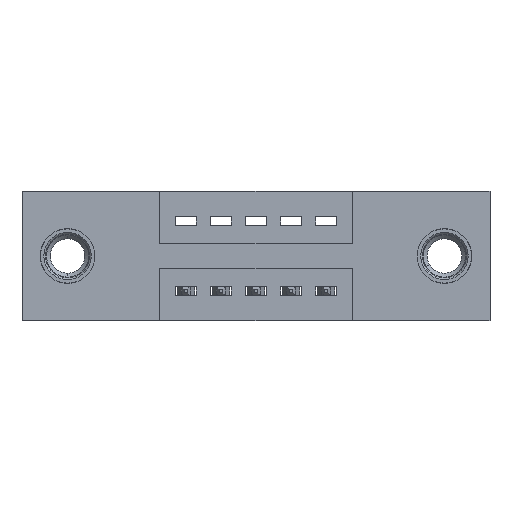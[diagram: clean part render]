
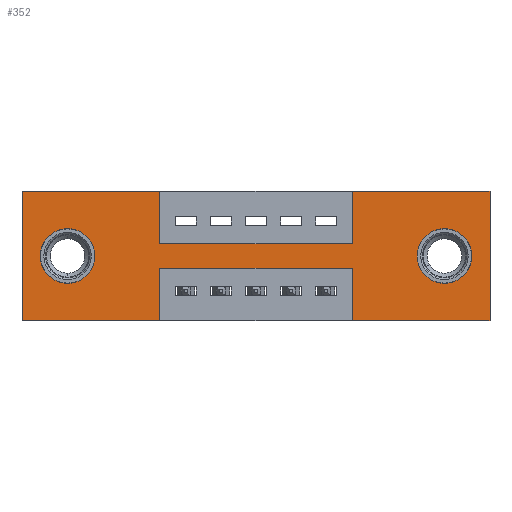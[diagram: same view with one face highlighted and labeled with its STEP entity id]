
A CAD part, front view. The second image highlights one B-rep face of the part: STEP entity #352.
In plain terms, the highlighted planar face has unit normal (0, -1, 0).
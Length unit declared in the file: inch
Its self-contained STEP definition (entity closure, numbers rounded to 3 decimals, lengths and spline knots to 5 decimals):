
#28 = VERTEX_POINT ( 'NONE', #2051 ) ;
#45 = CARTESIAN_POINT ( 'NONE',  ( 0.13, 0., -0.263 ) ) ;
#69 = ORIENTED_EDGE ( 'NONE', *, *, #4943, .F. ) ;
#73 = CARTESIAN_POINT ( 'NONE',  ( 0.3925, 0., -0.22 ) ) ;
#151 = VECTOR ( 'NONE', #3719, 39.37008 ) ;
#238 = CIRCLE ( 'NONE', #2748, 0.078 ) ;
#253 = VERTEX_POINT ( 'NONE', #2295 ) ;
#296 = CARTESIAN_POINT ( 'NONE',  ( 0.9425, 0., -0.37 ) ) ;
#352 = ADVANCED_FACE ( 'NONE', ( #1075, #2657, #8545 ), #2574, .T. ) ;
#358 = DIRECTION ( 'NONE',  ( 0., 0., -1. ) ) ;
#385 = VECTOR ( 'NONE', #1901, 39.37008 ) ;
#388 = VERTEX_POINT ( 'NONE', #4144 ) ;
#391 = DIRECTION ( 'NONE',  ( 0., 1., 0. ) ) ;
#530 = CARTESIAN_POINT ( 'NONE',  ( 0., 0., 0. ) ) ;
#558 = ORIENTED_EDGE ( 'NONE', *, *, #7253, .F. ) ;
#677 = VERTEX_POINT ( 'NONE', #1486 ) ;
#724 = LINE ( 'NONE', #1083, #8659 ) ;
#763 = VERTEX_POINT ( 'NONE', #45 ) ;
#806 = EDGE_CURVE ( 'NONE', #6764, #9784, #9596, .T. ) ;
#897 = CARTESIAN_POINT ( 'NONE',  ( 0.9425, 0., -0.15 ) ) ;
#1017 = DIRECTION ( 'NONE',  ( 0., 1., 0. ) ) ;
#1075 = FACE_BOUND ( 'NONE', #9132, .T. ) ;
#1083 = CARTESIAN_POINT ( 'NONE',  ( 1.335, 0., 0. ) ) ;
#1161 = ORIENTED_EDGE ( 'NONE', *, *, #9936, .F. ) ;
#1311 = VECTOR ( 'NONE', #2848, 39.37008 ) ;
#1486 = CARTESIAN_POINT ( 'NONE',  ( 1.205, 0., -0.107 ) ) ;
#1519 = ORIENTED_EDGE ( 'NONE', *, *, #2646, .F. ) ;
#1689 = LINE ( 'NONE', #6622, #5792 ) ;
#1882 = EDGE_LOOP ( 'NONE', ( #9166, #5014 ) ) ;
#1901 = DIRECTION ( 'NONE',  ( 1., 0., 0. ) ) ;
#1943 = LINE ( 'NONE', #9432, #7854 ) ;
#2003 = DIRECTION ( 'NONE',  ( 0., 0., 1. ) ) ;
#2026 = EDGE_CURVE ( 'NONE', #4399, #3299, #5590, .T. ) ;
#2037 = CARTESIAN_POINT ( 'NONE',  ( 0.3925, 0., -0.22 ) ) ;
#2051 = CARTESIAN_POINT ( 'NONE',  ( 0., 0., 0. ) ) ;
#2217 = LINE ( 'NONE', #296, #5832 ) ;
#2295 = CARTESIAN_POINT ( 'NONE',  ( 0.3925, 0., -0.15 ) ) ;
#2343 = VECTOR ( 'NONE', #5898, 39.37008 ) ;
#2426 = AXIS2_PLACEMENT_3D ( 'NONE', #8633, #4018, #9411 ) ;
#2428 = LINE ( 'NONE', #3425, #385 ) ;
#2490 = EDGE_CURVE ( 'NONE', #3299, #6764, #2217, .T. ) ;
#2574 = PLANE ( 'NONE',  #4707 ) ;
#2646 = EDGE_CURVE ( 'NONE', #6790, #7220, #8218, .T. ) ;
#2657 = FACE_BOUND ( 'NONE', #1882, .T. ) ;
#2668 = ORIENTED_EDGE ( 'NONE', *, *, #2026, .F. ) ;
#2745 = CARTESIAN_POINT ( 'NONE',  ( 0.9425, 0., -0.22 ) ) ;
#2748 = AXIS2_PLACEMENT_3D ( 'NONE', #4505, #9869, #5278 ) ;
#2848 = DIRECTION ( 'NONE',  ( -1., 0., 0. ) ) ;
#2850 = DIRECTION ( 'NONE',  ( -1., 0., 0. ) ) ;
#2927 = DIRECTION ( 'NONE',  ( -1., 0., 0. ) ) ;
#2999 = CIRCLE ( 'NONE', #9255, 0.078 ) ;
#3002 = EDGE_CURVE ( 'NONE', #763, #7161, #5111, .T. ) ;
#3026 = VECTOR ( 'NONE', #7493, 39.37008 ) ;
#3113 = ORIENTED_EDGE ( 'NONE', *, *, #4384, .F. ) ;
#3299 = VERTEX_POINT ( 'NONE', #9014 ) ;
#3335 = DIRECTION ( 'NONE',  ( 0., -1., 0. ) ) ;
#3425 = CARTESIAN_POINT ( 'NONE',  ( 0.3925, 0., -0.15 ) ) ;
#3529 = ORIENTED_EDGE ( 'NONE', *, *, #4447, .F. ) ;
#3543 = VECTOR ( 'NONE', #2927, 39.37008 ) ;
#3552 = CARTESIAN_POINT ( 'NONE',  ( 1.335, 0., -0.37 ) ) ;
#3719 = DIRECTION ( 'NONE',  ( 1., 0., 0. ) ) ;
#3785 = CARTESIAN_POINT ( 'NONE',  ( 0.3925, 0., -0.37 ) ) ;
#3820 = CARTESIAN_POINT ( 'NONE',  ( 0.3925, 0., 0. ) ) ;
#3893 = EDGE_CURVE ( 'NONE', #28, #5803, #8321, .T. ) ;
#3903 = AXIS2_PLACEMENT_3D ( 'NONE', #5621, #1017, #6402 ) ;
#3907 = ORIENTED_EDGE ( 'NONE', *, *, #3893, .F. ) ;
#4018 = DIRECTION ( 'NONE',  ( 0., 1., 0. ) ) ;
#4144 = CARTESIAN_POINT ( 'NONE',  ( 0.3925, 0., -0.37 ) ) ;
#4303 = EDGE_CURVE ( 'NONE', #253, #8958, #2428, .T. ) ;
#4384 = EDGE_CURVE ( 'NONE', #4739, #28, #1689, .T. ) ;
#4399 = VERTEX_POINT ( 'NONE', #3552 ) ;
#4447 = EDGE_CURVE ( 'NONE', #5803, #253, #5313, .T. ) ;
#4505 = CARTESIAN_POINT ( 'NONE',  ( 1.205, 0., -0.185 ) ) ;
#4508 = CARTESIAN_POINT ( 'NONE',  ( 0., 0., 0. ) ) ;
#4584 = DIRECTION ( 'NONE',  ( 0., 0., -1. ) ) ;
#4707 = AXIS2_PLACEMENT_3D ( 'NONE', #5623, #3335, #8718 ) ;
#4739 = VERTEX_POINT ( 'NONE', #5472 ) ;
#4776 = EDGE_LOOP ( 'NONE', ( #1161, #9934, #4787, #2668, #69, #1519, #558, #6356, #3529, #3907, #3113, #6937 ) ) ;
#4787 = ORIENTED_EDGE ( 'NONE', *, *, #2490, .F. ) ;
#4943 = EDGE_CURVE ( 'NONE', #7220, #4399, #724, .T. ) ;
#5004 = CARTESIAN_POINT ( 'NONE',  ( 1.205, 0., -0.185 ) ) ;
#5014 = ORIENTED_EDGE ( 'NONE', *, *, #3002, .T. ) ;
#5101 = EDGE_CURVE ( 'NONE', #388, #4739, #5413, .T. ) ;
#5111 = CIRCLE ( 'NONE', #3903, 0.078 ) ;
#5278 = DIRECTION ( 'NONE',  ( 0., 0., -1. ) ) ;
#5313 = LINE ( 'NONE', #9007, #3026 ) ;
#5413 = LINE ( 'NONE', #7448, #1311 ) ;
#5472 = CARTESIAN_POINT ( 'NONE',  ( 0., 0., -0.37 ) ) ;
#5590 = LINE ( 'NONE', #9813, #3543 ) ;
#5621 = CARTESIAN_POINT ( 'NONE',  ( 0.13, 0., -0.185 ) ) ;
#5623 = CARTESIAN_POINT ( 'NONE',  ( 0., 0., -0.37 ) ) ;
#5763 = DIRECTION ( 'NONE',  ( 0., 0., -1. ) ) ;
#5792 = VECTOR ( 'NONE', #2003, 39.37008 ) ;
#5803 = VERTEX_POINT ( 'NONE', #3820 ) ;
#5832 = VECTOR ( 'NONE', #9522, 39.37008 ) ;
#5898 = DIRECTION ( 'NONE',  ( 1., 0., 0. ) ) ;
#6062 = CARTESIAN_POINT ( 'NONE',  ( 1.205, 0., -0.263 ) ) ;
#6344 = DIRECTION ( 'NONE',  ( 0., 0., 1. ) ) ;
#6356 = ORIENTED_EDGE ( 'NONE', *, *, #4303, .F. ) ;
#6402 = DIRECTION ( 'NONE',  ( 0., 0., 1. ) ) ;
#6622 = CARTESIAN_POINT ( 'NONE',  ( 0., 0., 0. ) ) ;
#6764 = VERTEX_POINT ( 'NONE', #2745 ) ;
#6790 = VERTEX_POINT ( 'NONE', #7389 ) ;
#6937 = ORIENTED_EDGE ( 'NONE', *, *, #5101, .F. ) ;
#7161 = VERTEX_POINT ( 'NONE', #9328 ) ;
#7220 = VERTEX_POINT ( 'NONE', #7853 ) ;
#7253 = EDGE_CURVE ( 'NONE', #8958, #6790, #1943, .T. ) ;
#7389 = CARTESIAN_POINT ( 'NONE',  ( 0.9425, 0., 0. ) ) ;
#7448 = CARTESIAN_POINT ( 'NONE',  ( 0., 0., -0.37 ) ) ;
#7493 = DIRECTION ( 'NONE',  ( 0., 0., -1. ) ) ;
#7553 = VECTOR ( 'NONE', #2850, 39.37008 ) ;
#7703 = CIRCLE ( 'NONE', #2426, 0.078 ) ;
#7761 = LINE ( 'NONE', #3785, #9810 ) ;
#7853 = CARTESIAN_POINT ( 'NONE',  ( 1.335, 0., 0. ) ) ;
#7854 = VECTOR ( 'NONE', #6344, 39.37008 ) ;
#7965 = ORIENTED_EDGE ( 'NONE', *, *, #8771, .T. ) ;
#8218 = LINE ( 'NONE', #530, #2343 ) ;
#8321 = LINE ( 'NONE', #4508, #151 ) ;
#8345 = EDGE_CURVE ( 'NONE', #7161, #763, #7703, .T. ) ;
#8450 = ORIENTED_EDGE ( 'NONE', *, *, #9159, .T. ) ;
#8545 = FACE_OUTER_BOUND ( 'NONE', #4776, .T. ) ;
#8633 = CARTESIAN_POINT ( 'NONE',  ( 0.13, 0., -0.185 ) ) ;
#8659 = VECTOR ( 'NONE', #358, 39.37008 ) ;
#8718 = DIRECTION ( 'NONE',  ( 0., 0., -1. ) ) ;
#8771 = EDGE_CURVE ( 'NONE', #677, #9905, #238, .T. ) ;
#8958 = VERTEX_POINT ( 'NONE', #897 ) ;
#9007 = CARTESIAN_POINT ( 'NONE',  ( 0.3925, 0., 0. ) ) ;
#9014 = CARTESIAN_POINT ( 'NONE',  ( 0.9425, 0., -0.37 ) ) ;
#9132 = EDGE_LOOP ( 'NONE', ( #7965, #8450 ) ) ;
#9159 = EDGE_CURVE ( 'NONE', #9905, #677, #2999, .T. ) ;
#9166 = ORIENTED_EDGE ( 'NONE', *, *, #8345, .T. ) ;
#9255 = AXIS2_PLACEMENT_3D ( 'NONE', #5004, #391, #5763 ) ;
#9328 = CARTESIAN_POINT ( 'NONE',  ( 0.13, 0., -0.107 ) ) ;
#9411 = DIRECTION ( 'NONE',  ( 0., 0., 1. ) ) ;
#9432 = CARTESIAN_POINT ( 'NONE',  ( 0.9425, 0., 0. ) ) ;
#9522 = DIRECTION ( 'NONE',  ( 0., 0., 1. ) ) ;
#9596 = LINE ( 'NONE', #73, #7553 ) ;
#9784 = VERTEX_POINT ( 'NONE', #2037 ) ;
#9810 = VECTOR ( 'NONE', #4584, 39.37008 ) ;
#9813 = CARTESIAN_POINT ( 'NONE',  ( 0., 0., -0.37 ) ) ;
#9869 = DIRECTION ( 'NONE',  ( 0., 1., 0. ) ) ;
#9905 = VERTEX_POINT ( 'NONE', #6062 ) ;
#9934 = ORIENTED_EDGE ( 'NONE', *, *, #806, .F. ) ;
#9936 = EDGE_CURVE ( 'NONE', #9784, #388, #7761, .T. ) ;
